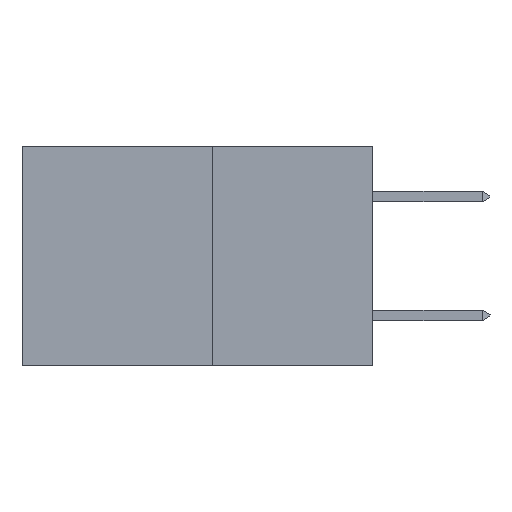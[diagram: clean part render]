
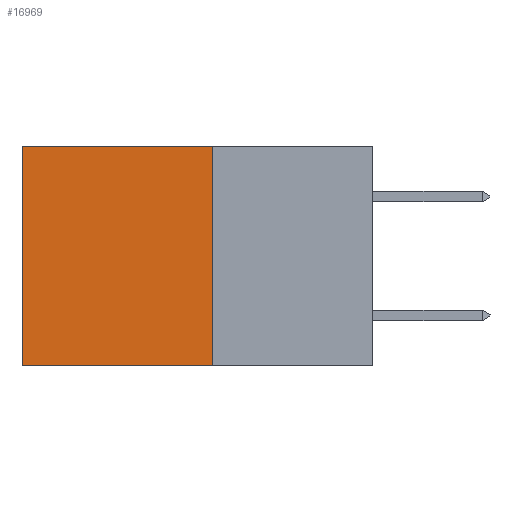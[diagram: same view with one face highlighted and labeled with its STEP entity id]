
A CAD part, left-side view. The second image highlights one B-rep face of the part: STEP entity #16969.
In plain terms, the highlighted planar face has unit normal (-1, 0, 0).
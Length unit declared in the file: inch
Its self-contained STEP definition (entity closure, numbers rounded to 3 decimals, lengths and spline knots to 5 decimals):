
#347 = ORIENTED_EDGE ( 'NONE', *, *, #20020, .F. ) ;
#405 = LINE ( 'NONE', #11642, #4486 ) ;
#845 = DIRECTION ( 'NONE',  ( 0., 0., -1. ) ) ;
#1383 = CARTESIAN_POINT ( 'NONE',  ( 0.277, 0.27, -0.37 ) ) ;
#2888 = VERTEX_POINT ( 'NONE', #13912 ) ;
#3447 = LINE ( 'NONE', #17124, #8123 ) ;
#3726 = DIRECTION ( 'NONE',  ( 0., 0., -1. ) ) ;
#4486 = VECTOR ( 'NONE', #3726, 39.37008 ) ;
#5712 = EDGE_CURVE ( 'NONE', #2888, #22265, #10949, .T. ) ;
#6786 = CARTESIAN_POINT ( 'NONE',  ( 0.277, 0.27, -0.37 ) ) ;
#6895 = LINE ( 'NONE', #8421, #10915 ) ;
#8123 = VECTOR ( 'NONE', #19167, 39.37008 ) ;
#8421 = CARTESIAN_POINT ( 'NONE',  ( 0.277, 0.27, -0.37 ) ) ;
#8474 = ORIENTED_EDGE ( 'NONE', *, *, #11192, .T. ) ;
#8707 = ORIENTED_EDGE ( 'NONE', *, *, #16207, .F. ) ;
#8710 = FACE_OUTER_BOUND ( 'NONE', #25187, .T. ) ;
#10915 = VECTOR ( 'NONE', #20282, 39.37008 ) ;
#10949 = LINE ( 'NONE', #21272, #20263 ) ;
#11192 = EDGE_CURVE ( 'NONE', #22265, #23190, #405, .T. ) ;
#11642 = CARTESIAN_POINT ( 'NONE',  ( 0.277, 0.59, -0.37 ) ) ;
#12673 = PLANE ( 'NONE',  #13354 ) ;
#12758 = DIRECTION ( 'NONE',  ( 1., 0., 0. ) ) ;
#12807 = CARTESIAN_POINT ( 'NONE',  ( 0.277, 0.59, -0.37 ) ) ;
#13354 = AXIS2_PLACEMENT_3D ( 'NONE', #6786, #12758, #845 ) ;
#13397 = DIRECTION ( 'NONE',  ( 0., 1., 0. ) ) ;
#13785 = CARTESIAN_POINT ( 'NONE',  ( 0.277, 0.59, 0. ) ) ;
#13878 = VERTEX_POINT ( 'NONE', #1383 ) ;
#13912 = CARTESIAN_POINT ( 'NONE',  ( 0.277, 0.27, 0. ) ) ;
#15120 = ORIENTED_EDGE ( 'NONE', *, *, #5712, .T. ) ;
#16207 = EDGE_CURVE ( 'NONE', #13878, #23190, #6895, .T. ) ;
#16969 = ADVANCED_FACE ( 'NONE', ( #8710 ), #12673, .F. ) ;
#17124 = CARTESIAN_POINT ( 'NONE',  ( 0.277, 0.27, -0.37 ) ) ;
#19167 = DIRECTION ( 'NONE',  ( 0., 0., -1. ) ) ;
#20020 = EDGE_CURVE ( 'NONE', #2888, #13878, #3447, .T. ) ;
#20263 = VECTOR ( 'NONE', #13397, 39.37008 ) ;
#20282 = DIRECTION ( 'NONE',  ( 0., 1., 0. ) ) ;
#21272 = CARTESIAN_POINT ( 'NONE',  ( 0.277, 0.27, 0. ) ) ;
#22265 = VERTEX_POINT ( 'NONE', #13785 ) ;
#23190 = VERTEX_POINT ( 'NONE', #12807 ) ;
#25187 = EDGE_LOOP ( 'NONE', ( #8474, #8707, #347, #15120 ) ) ;
